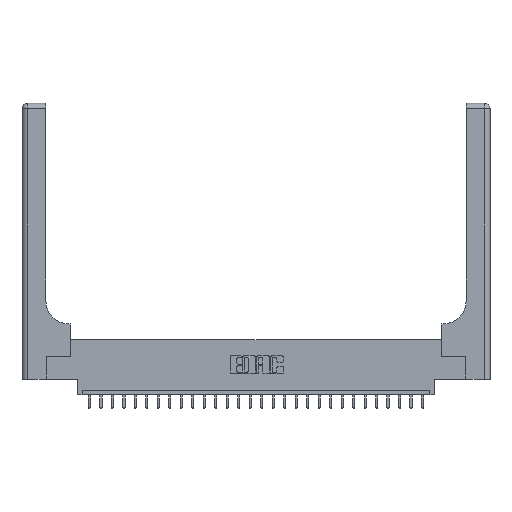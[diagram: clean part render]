
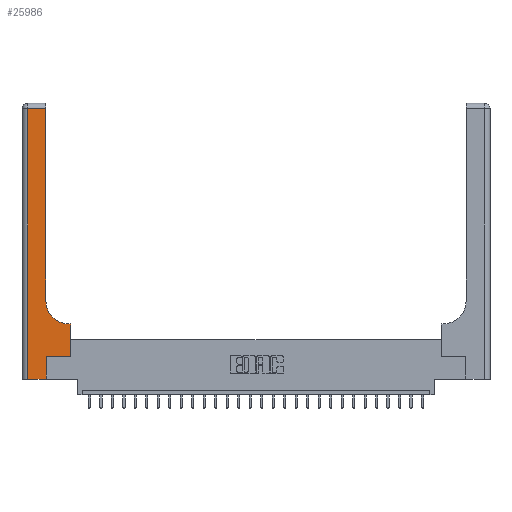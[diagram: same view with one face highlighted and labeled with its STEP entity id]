
A CAD part, top view. The second image highlights one B-rep face of the part: STEP entity #25986.
In plain terms, the highlighted planar face has unit normal (0, 0, 1).
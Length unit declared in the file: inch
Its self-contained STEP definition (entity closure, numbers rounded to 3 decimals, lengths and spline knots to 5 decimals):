
#445 = VECTOR ( 'NONE', #17966, 39.37008 ) ;
#1212 = CARTESIAN_POINT ( 'NONE',  ( 0.06, 2.94, 0.37 ) ) ;
#1455 = VERTEX_POINT ( 'NONE', #4187 ) ;
#2265 = VERTEX_POINT ( 'NONE', #17880 ) ;
#2315 = VECTOR ( 'NONE', #4491, 39.37008 ) ;
#2382 = LINE ( 'NONE', #10290, #2315 ) ;
#3247 = EDGE_CURVE ( 'NONE', #3531, #1455, #16824, .T. ) ;
#3531 = VERTEX_POINT ( 'NONE', #9389 ) ;
#3650 = ORIENTED_EDGE ( 'NONE', *, *, #9419, .T. ) ;
#3766 = VECTOR ( 'NONE', #17869, 39.37008 ) ;
#4080 = ORIENTED_EDGE ( 'NONE', *, *, #17817, .T. ) ;
#4187 = CARTESIAN_POINT ( 'NONE',  ( 0.26, 0.85, 0.37 ) ) ;
#4279 = LINE ( 'NONE', #24140, #445 ) ;
#4413 = EDGE_CURVE ( 'NONE', #23585, #21357, #20425, .T. ) ;
#4426 = VECTOR ( 'NONE', #5572, 39.37008 ) ;
#4491 = DIRECTION ( 'NONE',  ( 0., 1., 0. ) ) ;
#4648 = CARTESIAN_POINT ( 'NONE',  ( 0., 0., 0.37 ) ) ;
#5572 = DIRECTION ( 'NONE',  ( 0., 1., 0. ) ) ;
#6345 = DIRECTION ( 'NONE',  ( 1., 0., 0. ) ) ;
#7414 = CARTESIAN_POINT ( 'NONE',  ( 0.26, 3., 0.37 ) ) ;
#7529 = DIRECTION ( 'NONE',  ( -1., 0., 0. ) ) ;
#7957 = DIRECTION ( 'NONE',  ( 1., 0., 0. ) ) ;
#8195 = LINE ( 'NONE', #24119, #25187 ) ;
#8658 = ORIENTED_EDGE ( 'NONE', *, *, #25143, .T. ) ;
#9389 = CARTESIAN_POINT ( 'NONE',  ( 0.51, 0.6, 0.37 ) ) ;
#9419 = EDGE_CURVE ( 'NONE', #13629, #21361, #9890, .T. ) ;
#9890 = LINE ( 'NONE', #13716, #10069 ) ;
#10047 = ORIENTED_EDGE ( 'NONE', *, *, #17516, .T. ) ;
#10069 = VECTOR ( 'NONE', #13592, 39.37008 ) ;
#10290 = CARTESIAN_POINT ( 'NONE',  ( 0.265, 0., 0.37 ) ) ;
#12438 = DIRECTION ( 'NONE',  ( 1., 0., 0. ) ) ;
#12842 = CARTESIAN_POINT ( 'NONE',  ( 0.265, 0.25, 0.37 ) ) ;
#12989 = VERTEX_POINT ( 'NONE', #1212 ) ;
#13592 = DIRECTION ( 'NONE',  ( 0., 1., 0. ) ) ;
#13627 = CARTESIAN_POINT ( 'NONE',  ( 0.51, 0.85, 0.37 ) ) ;
#13629 = VERTEX_POINT ( 'NONE', #16319 ) ;
#13672 = LINE ( 'NONE', #19953, #3766 ) ;
#13716 = CARTESIAN_POINT ( 'NONE',  ( 0.528, 0.25, 0.37 ) ) ;
#13819 = ORIENTED_EDGE ( 'NONE', *, *, #14528, .T. ) ;
#13854 = ORIENTED_EDGE ( 'NONE', *, *, #22508, .T. ) ;
#14080 = DIRECTION ( 'NONE',  ( -1., 0., 0. ) ) ;
#14528 = EDGE_CURVE ( 'NONE', #12989, #23585, #4279, .T. ) ;
#14670 = VERTEX_POINT ( 'NONE', #12842 ) ;
#14923 = CARTESIAN_POINT ( 'NONE',  ( 0.528, 0.6, 0.37 ) ) ;
#15323 = CARTESIAN_POINT ( 'NONE',  ( 0.265, 0., 0.37 ) ) ;
#16319 = CARTESIAN_POINT ( 'NONE',  ( 0.528, 0.25, 0.37 ) ) ;
#16571 = ORIENTED_EDGE ( 'NONE', *, *, #3247, .T. ) ;
#16638 = EDGE_LOOP ( 'NONE', ( #18934, #13854, #13819, #24341, #8658, #10047, #3650, #4080, #16571 ) ) ;
#16824 = CIRCLE ( 'NONE', #21443, 0.25 ) ;
#17516 = EDGE_CURVE ( 'NONE', #14670, #13629, #8195, .T. ) ;
#17817 = EDGE_CURVE ( 'NONE', #21361, #3531, #13672, .T. ) ;
#17869 = DIRECTION ( 'NONE',  ( -1., 0., 0. ) ) ;
#17880 = CARTESIAN_POINT ( 'NONE',  ( 0.26, 2.94, 0.37 ) ) ;
#17941 = LINE ( 'NONE', #7414, #4426 ) ;
#17966 = DIRECTION ( 'NONE',  ( 0., -1., 0. ) ) ;
#18016 = LINE ( 'NONE', #19970, #21543 ) ;
#18934 = ORIENTED_EDGE ( 'NONE', *, *, #19751, .T. ) ;
#19373 = FACE_OUTER_BOUND ( 'NONE', #16638, .T. ) ;
#19751 = EDGE_CURVE ( 'NONE', #1455, #2265, #17941, .T. ) ;
#19953 = CARTESIAN_POINT ( 'NONE',  ( 0.26, 0.6, 0.37 ) ) ;
#19970 = CARTESIAN_POINT ( 'NONE',  ( 0., 2.94, 0.37 ) ) ;
#20425 = LINE ( 'NONE', #4648, #23181 ) ;
#21351 = PLANE ( 'NONE',  #22932 ) ;
#21357 = VERTEX_POINT ( 'NONE', #15323 ) ;
#21361 = VERTEX_POINT ( 'NONE', #14923 ) ;
#21443 = AXIS2_PLACEMENT_3D ( 'NONE', #13627, #25983, #7957 ) ;
#21543 = VECTOR ( 'NONE', #14080, 39.37008 ) ;
#22508 = EDGE_CURVE ( 'NONE', #2265, #12989, #18016, .T. ) ;
#22932 = AXIS2_PLACEMENT_3D ( 'NONE', #25182, #25576, #7529 ) ;
#23181 = VECTOR ( 'NONE', #12438, 39.37008 ) ;
#23585 = VERTEX_POINT ( 'NONE', #24262 ) ;
#24119 = CARTESIAN_POINT ( 'NONE',  ( 0.265, 0.25, 0.37 ) ) ;
#24140 = CARTESIAN_POINT ( 'NONE',  ( 0.06, 3., 0.37 ) ) ;
#24262 = CARTESIAN_POINT ( 'NONE',  ( 0.06, 0., 0.37 ) ) ;
#24341 = ORIENTED_EDGE ( 'NONE', *, *, #4413, .T. ) ;
#25143 = EDGE_CURVE ( 'NONE', #21357, #14670, #2382, .T. ) ;
#25182 = CARTESIAN_POINT ( 'NONE',  ( 0., 3., 0.37 ) ) ;
#25187 = VECTOR ( 'NONE', #6345, 39.37008 ) ;
#25576 = DIRECTION ( 'NONE',  ( 0., 0., -1. ) ) ;
#25983 = DIRECTION ( 'NONE',  ( 0., 0., -1. ) ) ;
#25986 = ADVANCED_FACE ( 'NONE', ( #19373 ), #21351, .F. ) ;
